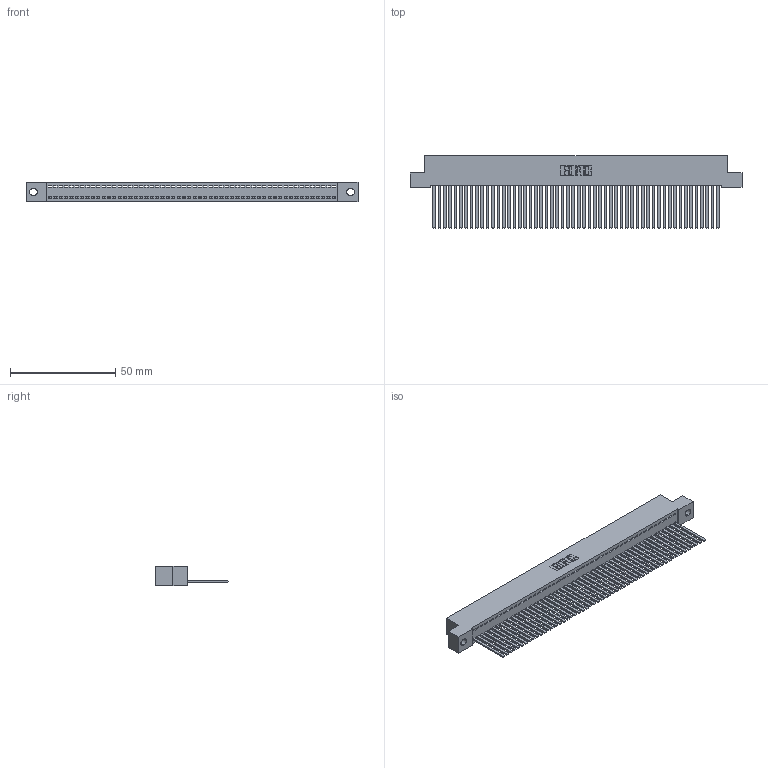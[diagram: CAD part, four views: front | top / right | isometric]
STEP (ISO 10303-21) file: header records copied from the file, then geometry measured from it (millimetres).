
FILE_DESCRIPTION (( 'STEP AP203' ), '1' );
FILE_NAME ('392-054-544-102.STEP', '2019-10-08T13:57:07', ( '' ), ( '' ), 'SwSTEP 2.0', 'SolidWorks 2016', '' );
FILE_SCHEMA (( 'CONFIG_CONTROL_DESIGN' ));
Length unit declared in the file: inch
Products named in the file (3): 342 Part_.128 Slot; 345-292-001_345-293-144; 392-054-544-102
Assembly tree (55 placements, depth 2):
  392-054-544-102
    342 Part_.128 Slot
    345-292-001_345-293-144  x54
Bounding box: 157.48 x 34.3 x 9.4 mm (x, y, z)
Volume: 14425.3 mm3; surface area: 22946.5 mm2
Topology: 55 solids, 55 shells, 2922 faces, 8843 edges, 5822 vertices
Faces by surface type: plane 2122, cylinder 800
Entity records: 31279 total; most frequent: CARTESIAN_POINT 5400, ORIENTED_EDGE 5390, DIRECTION 4527, EDGE_CURVE 2695, LINE 2571, VECTOR 2571, VERTEX_POINT 1794, AXIS2_PLACEMENT_3D 978
